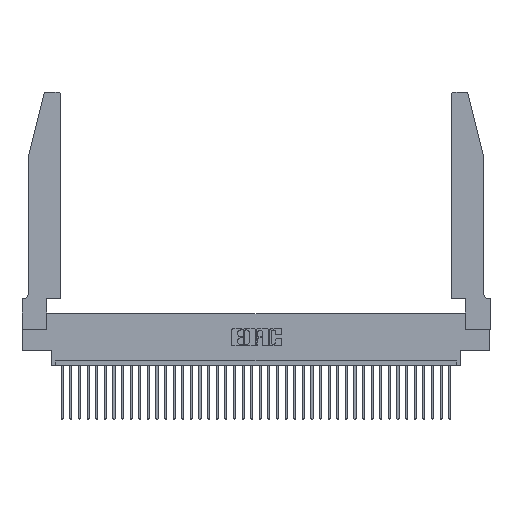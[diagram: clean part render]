
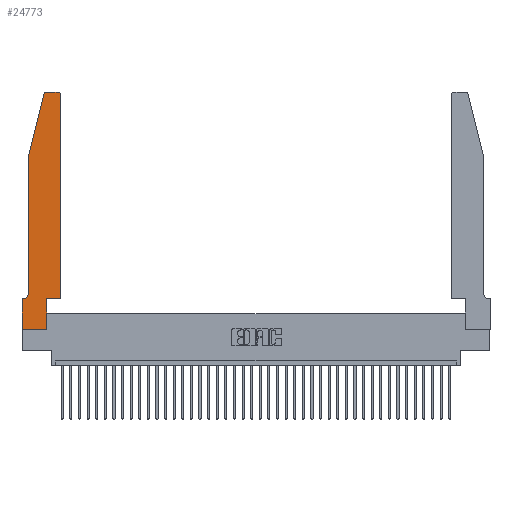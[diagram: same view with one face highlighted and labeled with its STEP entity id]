
A CAD part, top view. The second image highlights one B-rep face of the part: STEP entity #24773.
In plain terms, the highlighted planar face has unit normal (0, 0, 1).
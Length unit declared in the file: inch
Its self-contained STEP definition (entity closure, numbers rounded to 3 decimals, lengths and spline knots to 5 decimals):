
#32 = DIRECTION ( 'NONE',  ( 0., 0., 1. ) ) ;
#634 = VECTOR ( 'NONE', #38406, 39.37008 ) ;
#992 = AXIS2_PLACEMENT_3D ( 'NONE', #1548, #7319, #22583 ) ;
#1102 = VERTEX_POINT ( 'NONE', #14312 ) ;
#1396 = ORIENTED_EDGE ( 'NONE', *, *, #32735, .T. ) ;
#1548 = CARTESIAN_POINT ( 'NONE',  ( 0.284, 2.72, 0.37 ) ) ;
#1712 = LINE ( 'NONE', #32398, #30349 ) ;
#2028 = VECTOR ( 'NONE', #6504, 39.37008 ) ;
#3048 = VERTEX_POINT ( 'NONE', #18646 ) ;
#3243 = VERTEX_POINT ( 'NONE', #27590 ) ;
#3317 = VERTEX_POINT ( 'NONE', #18292 ) ;
#4273 = DIRECTION ( 'NONE',  ( 0., -1., 0. ) ) ;
#4533 = LINE ( 'NONE', #17657, #19607 ) ;
#4626 = VECTOR ( 'NONE', #32695, 39.37008 ) ;
#5313 = DIRECTION ( 'NONE',  ( 1., 0., 0. ) ) ;
#5412 = EDGE_CURVE ( 'NONE', #3048, #3243, #17625, .T. ) ;
#5699 = EDGE_CURVE ( 'NONE', #38897, #22345, #16739, .T. ) ;
#5879 = AXIS2_PLACEMENT_3D ( 'NONE', #13571, #37640, #7518 ) ;
#5900 = LINE ( 'NONE', #22293, #36929 ) ;
#6081 = EDGE_CURVE ( 'NONE', #1102, #35494, #5900, .T. ) ;
#6504 = DIRECTION ( 'NONE',  ( -1., 0., 0. ) ) ;
#6569 = PLANE ( 'NONE',  #18280 ) ;
#7285 = DIRECTION ( 'NONE',  ( 0., 1., 0. ) ) ;
#7315 = ORIENTED_EDGE ( 'NONE', *, *, #29190, .T. ) ;
#7319 = DIRECTION ( 'NONE',  ( 0., 0., 1. ) ) ;
#7518 = DIRECTION ( 'NONE',  ( -1., 0., 0. ) ) ;
#8022 = CARTESIAN_POINT ( 'NONE',  ( 0.0755, 2., 0.37 ) ) ;
#8373 = VERTEX_POINT ( 'NONE', #32095 ) ;
#8482 = CARTESIAN_POINT ( 'NONE',  ( 0.4205, 2.72, 0.37 ) ) ;
#9126 = DIRECTION ( 'NONE',  ( 1., 0., 0. ) ) ;
#9510 = ORIENTED_EDGE ( 'NONE', *, *, #14419, .T. ) ;
#9988 = LINE ( 'NONE', #17924, #2028 ) ;
#10193 = VERTEX_POINT ( 'NONE', #20886 ) ;
#10543 = EDGE_CURVE ( 'NONE', #3243, #1102, #25333, .T. ) ;
#11974 = FACE_OUTER_BOUND ( 'NONE', #20719, .T. ) ;
#13029 = LINE ( 'NONE', #24929, #36135 ) ;
#13571 = CARTESIAN_POINT ( 'NONE',  ( 0.0055, 0.42, 0.37 ) ) ;
#14312 = CARTESIAN_POINT ( 'NONE',  ( 0., 0.35, 0.37 ) ) ;
#14370 = DIRECTION ( 'NONE',  ( -0.239, -0.971, 0. ) ) ;
#14419 = EDGE_CURVE ( 'NONE', #27676, #8373, #9988, .T. ) ;
#14534 = DIRECTION ( 'NONE',  ( 0., 0., 1. ) ) ;
#14578 = CARTESIAN_POINT ( 'NONE',  ( 0.4205, 2.75, 0.37 ) ) ;
#16669 = CARTESIAN_POINT ( 'NONE',  ( 0.4505, 0.35, 0.37 ) ) ;
#16739 = LINE ( 'NONE', #31693, #634 ) ;
#17019 = ORIENTED_EDGE ( 'NONE', *, *, #35757, .T. ) ;
#17216 = CARTESIAN_POINT ( 'NONE',  ( 0.0755, 0.35, 0.37 ) ) ;
#17625 = CIRCLE ( 'NONE', #5879, 0.07 ) ;
#17657 = CARTESIAN_POINT ( 'NONE',  ( 0., 0., 0.37 ) ) ;
#17924 = CARTESIAN_POINT ( 'NONE',  ( 0.2605, 2.75, 0.37 ) ) ;
#18066 = CARTESIAN_POINT ( 'NONE',  ( 0., 0.35, 0.37 ) ) ;
#18280 = AXIS2_PLACEMENT_3D ( 'NONE', #18066, #32, #9126 ) ;
#18292 = CARTESIAN_POINT ( 'NONE',  ( 0.4505, 2.72, 0.37 ) ) ;
#18646 = CARTESIAN_POINT ( 'NONE',  ( 0.0755, 0.42, 0.37 ) ) ;
#19044 = DIRECTION ( 'NONE',  ( 0., -1., 0. ) ) ;
#19607 = VECTOR ( 'NONE', #26359, 39.37008 ) ;
#20719 = EDGE_LOOP ( 'NONE', ( #9510, #28395, #1396, #37799, #21971, #20795, #24095, #7315, #37338, #34177, #31065, #17019 ) ) ;
#20795 = ORIENTED_EDGE ( 'NONE', *, *, #10543, .T. ) ;
#20875 = EDGE_CURVE ( 'NONE', #8373, #27311, #28359, .T. ) ;
#20886 = CARTESIAN_POINT ( 'NONE',  ( 0.4505, 0.35, 0.37 ) ) ;
#21901 = VECTOR ( 'NONE', #7285, 39.37008 ) ;
#21971 = ORIENTED_EDGE ( 'NONE', *, *, #5412, .T. ) ;
#22293 = CARTESIAN_POINT ( 'NONE',  ( 0., 0., 0.37 ) ) ;
#22345 = VERTEX_POINT ( 'NONE', #31224 ) ;
#22494 = VERTEX_POINT ( 'NONE', #8022 ) ;
#22583 = DIRECTION ( 'NONE',  ( 1., 0., 0. ) ) ;
#22656 = LINE ( 'NONE', #35594, #38675 ) ;
#23506 = EDGE_CURVE ( 'NONE', #22494, #3048, #13029, .T. ) ;
#24095 = ORIENTED_EDGE ( 'NONE', *, *, #6081, .T. ) ;
#24764 = AXIS2_PLACEMENT_3D ( 'NONE', #8482, #14534, #38847 ) ;
#24773 = ADVANCED_FACE ( 'NONE', ( #11974 ), #6569, .T. ) ;
#24929 = CARTESIAN_POINT ( 'NONE',  ( 0.0755, 2., 0.37 ) ) ;
#25333 = LINE ( 'NONE', #17216, #4626 ) ;
#26359 = DIRECTION ( 'NONE',  ( 1., 0., 0. ) ) ;
#26439 = EDGE_CURVE ( 'NONE', #22345, #10193, #22656, .T. ) ;
#27311 = VERTEX_POINT ( 'NONE', #36049 ) ;
#27590 = CARTESIAN_POINT ( 'NONE',  ( 0.0055, 0.35, 0.37 ) ) ;
#27676 = VERTEX_POINT ( 'NONE', #14578 ) ;
#28359 = CIRCLE ( 'NONE', #992, 0.03 ) ;
#28395 = ORIENTED_EDGE ( 'NONE', *, *, #20875, .T. ) ;
#29190 = EDGE_CURVE ( 'NONE', #35494, #38897, #4533, .T. ) ;
#30069 = EDGE_CURVE ( 'NONE', #10193, #3317, #34155, .T. ) ;
#30349 = VECTOR ( 'NONE', #14370, 39.37008 ) ;
#31065 = ORIENTED_EDGE ( 'NONE', *, *, #30069, .T. ) ;
#31224 = CARTESIAN_POINT ( 'NONE',  ( 0.2865, 0.35, 0.37 ) ) ;
#31693 = CARTESIAN_POINT ( 'NONE',  ( 0.2865, 0.35, 0.37 ) ) ;
#32095 = CARTESIAN_POINT ( 'NONE',  ( 0.284, 2.75, 0.37 ) ) ;
#32166 = CARTESIAN_POINT ( 'NONE',  ( 0., 0., 0.37 ) ) ;
#32398 = CARTESIAN_POINT ( 'NONE',  ( 0.0755, 2., 0.37 ) ) ;
#32695 = DIRECTION ( 'NONE',  ( -1., 0., 0. ) ) ;
#32735 = EDGE_CURVE ( 'NONE', #27311, #22494, #1712, .T. ) ;
#33440 = CIRCLE ( 'NONE', #24764, 0.03 ) ;
#34155 = LINE ( 'NONE', #16669, #21901 ) ;
#34177 = ORIENTED_EDGE ( 'NONE', *, *, #26439, .T. ) ;
#35494 = VERTEX_POINT ( 'NONE', #32166 ) ;
#35594 = CARTESIAN_POINT ( 'NONE',  ( 0.4505, 0.35, 0.37 ) ) ;
#35757 = EDGE_CURVE ( 'NONE', #3317, #27676, #33440, .T. ) ;
#36049 = CARTESIAN_POINT ( 'NONE',  ( 0.25487, 2.72718, 0.37 ) ) ;
#36135 = VECTOR ( 'NONE', #19044, 39.37008 ) ;
#36154 = CARTESIAN_POINT ( 'NONE',  ( 0.2865, 0., 0.37 ) ) ;
#36929 = VECTOR ( 'NONE', #4273, 39.37008 ) ;
#37338 = ORIENTED_EDGE ( 'NONE', *, *, #5699, .T. ) ;
#37640 = DIRECTION ( 'NONE',  ( 0., 0., -1. ) ) ;
#37799 = ORIENTED_EDGE ( 'NONE', *, *, #23506, .T. ) ;
#38406 = DIRECTION ( 'NONE',  ( 0., 1., 0. ) ) ;
#38675 = VECTOR ( 'NONE', #5313, 39.37008 ) ;
#38847 = DIRECTION ( 'NONE',  ( 1., 0., 0. ) ) ;
#38897 = VERTEX_POINT ( 'NONE', #36154 ) ;
